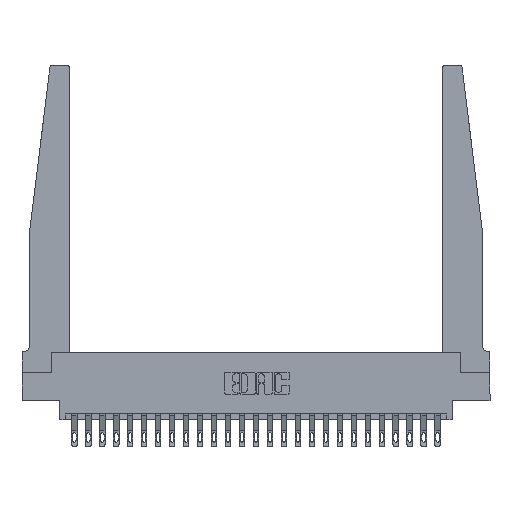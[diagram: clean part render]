
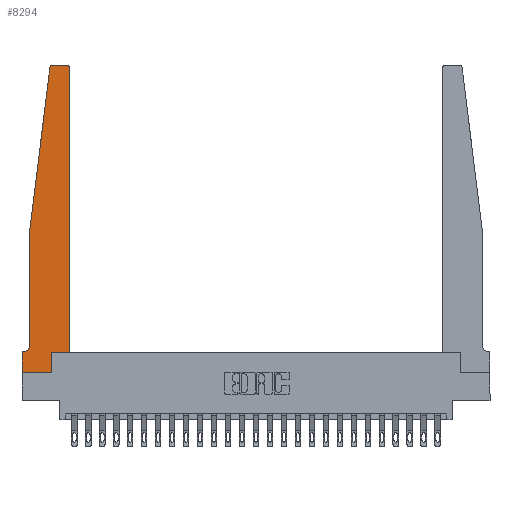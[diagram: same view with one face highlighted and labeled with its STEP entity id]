
A CAD part, top view. The second image highlights one B-rep face of the part: STEP entity #8294.
In plain terms, the highlighted planar face has unit normal (0, 0, 1).
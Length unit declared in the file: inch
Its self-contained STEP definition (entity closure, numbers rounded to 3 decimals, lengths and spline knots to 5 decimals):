
#304 = DIRECTION ( 'NONE',  ( 1., 0., 0. ) ) ;
#438 = CARTESIAN_POINT ( 'NONE',  ( 0.425, 0.18, 0.37 ) ) ;
#448 = DIRECTION ( 'NONE',  ( 1., 0., 0. ) ) ;
#450 = CARTESIAN_POINT ( 'NONE',  ( 0.065, 1.25, 0.37 ) ) ;
#496 = LINE ( 'NONE', #16148, #21478 ) ;
#976 = LINE ( 'NONE', #18656, #2612 ) ;
#987 = VERTEX_POINT ( 'NONE', #24516 ) ;
#1313 = CARTESIAN_POINT ( 'NONE',  ( 0., 0., 0.37 ) ) ;
#1725 = AXIS2_PLACEMENT_3D ( 'NONE', #16326, #2731, #22064 ) ;
#1977 = EDGE_CURVE ( 'NONE', #16019, #15077, #976, .T. ) ;
#2506 = ORIENTED_EDGE ( 'NONE', *, *, #14173, .T. ) ;
#2612 = VECTOR ( 'NONE', #22486, 39.37008 ) ;
#2731 = DIRECTION ( 'NONE',  ( 0., 0., -1. ) ) ;
#3103 = VERTEX_POINT ( 'NONE', #23181 ) ;
#3325 = CARTESIAN_POINT ( 'NONE',  ( 0.065, 1.25, 0.37 ) ) ;
#4118 = AXIS2_PLACEMENT_3D ( 'NONE', #18171, #18535, #14461 ) ;
#4523 = EDGE_CURVE ( 'NONE', #987, #17057, #13668, .T. ) ;
#4649 = VERTEX_POINT ( 'NONE', #15840 ) ;
#4900 = AXIS2_PLACEMENT_3D ( 'NONE', #19414, #17512, #448 ) ;
#5252 = EDGE_CURVE ( 'NONE', #9253, #4649, #19997, .T. ) ;
#5402 = DIRECTION ( 'NONE',  ( -1., 0., 0. ) ) ;
#5615 = DIRECTION ( 'NONE',  ( 1., 0., 0. ) ) ;
#5643 = VERTEX_POINT ( 'NONE', #18322 ) ;
#6021 = ORIENTED_EDGE ( 'NONE', *, *, #4523, .T. ) ;
#6330 = VERTEX_POINT ( 'NONE', #450 ) ;
#6332 = ORIENTED_EDGE ( 'NONE', *, *, #1977, .T. ) ;
#6504 = EDGE_CURVE ( 'NONE', #3103, #10384, #11572, .T. ) ;
#6585 = AXIS2_PLACEMENT_3D ( 'NONE', #7555, #23144, #5615 ) ;
#6631 = ORIENTED_EDGE ( 'NONE', *, *, #19101, .T. ) ;
#6882 = VECTOR ( 'NONE', #19458, 39.37008 ) ;
#7091 = ORIENTED_EDGE ( 'NONE', *, *, #15475, .T. ) ;
#7186 = CARTESIAN_POINT ( 'NONE',  ( 0.425, 0.18, 0.37 ) ) ;
#7555 = CARTESIAN_POINT ( 'NONE',  ( 0.27653, 2.72, 0.37 ) ) ;
#8294 = ADVANCED_FACE ( 'NONE', ( #16136 ), #12296, .T. ) ;
#8692 = CIRCLE ( 'NONE', #1725, 0.05 ) ;
#9253 = VERTEX_POINT ( 'NONE', #22401 ) ;
#9381 = ORIENTED_EDGE ( 'NONE', *, *, #5252, .T. ) ;
#9398 = EDGE_CURVE ( 'NONE', #11589, #6330, #13097, .T. ) ;
#9650 = VECTOR ( 'NONE', #22900, 39.37008 ) ;
#10173 = ORIENTED_EDGE ( 'NONE', *, *, #10386, .T. ) ;
#10384 = VERTEX_POINT ( 'NONE', #14288 ) ;
#10386 = EDGE_CURVE ( 'NONE', #5643, #9253, #8692, .T. ) ;
#10797 = ORIENTED_EDGE ( 'NONE', *, *, #9398, .T. ) ;
#11281 = VECTOR ( 'NONE', #17853, 39.37008 ) ;
#11572 = LINE ( 'NONE', #15533, #25183 ) ;
#11589 = VERTEX_POINT ( 'NONE', #11617 ) ;
#11617 = CARTESIAN_POINT ( 'NONE',  ( 0.24675, 2.72367, 0.37 ) ) ;
#12296 = PLANE ( 'NONE',  #4118 ) ;
#12999 = ORIENTED_EDGE ( 'NONE', *, *, #25140, .T. ) ;
#13097 = LINE ( 'NONE', #3325, #6882 ) ;
#13668 = LINE ( 'NONE', #7186, #9650 ) ;
#14169 = LINE ( 'NONE', #438, #25206 ) ;
#14173 = EDGE_CURVE ( 'NONE', #17680, #16019, #496, .T. ) ;
#14231 = DIRECTION ( 'NONE',  ( 1., 0., 0. ) ) ;
#14264 = DIRECTION ( 'NONE',  ( 0., -1., 0. ) ) ;
#14288 = CARTESIAN_POINT ( 'NONE',  ( 0.27653, 2.75, 0.37 ) ) ;
#14461 = DIRECTION ( 'NONE',  ( 1., 0., 0. ) ) ;
#14935 = EDGE_CURVE ( 'NONE', #15077, #987, #14169, .T. ) ;
#15077 = VERTEX_POINT ( 'NONE', #16584 ) ;
#15475 = EDGE_CURVE ( 'NONE', #6330, #5643, #17604, .T. ) ;
#15533 = CARTESIAN_POINT ( 'NONE',  ( 0.25, 2.75, 0.37 ) ) ;
#15551 = CARTESIAN_POINT ( 'NONE',  ( 0.065, 1.25, 0.37 ) ) ;
#15803 = CARTESIAN_POINT ( 'NONE',  ( 0., 0., 0.37 ) ) ;
#15840 = CARTESIAN_POINT ( 'NONE',  ( 0., 0.1875, 0.37 ) ) ;
#16019 = VERTEX_POINT ( 'NONE', #24544 ) ;
#16136 = FACE_OUTER_BOUND ( 'NONE', #17041, .T. ) ;
#16148 = CARTESIAN_POINT ( 'NONE',  ( 0., 0., 0.37 ) ) ;
#16183 = LINE ( 'NONE', #15803, #18735 ) ;
#16193 = DIRECTION ( 'NONE',  ( -1., 0., 0. ) ) ;
#16326 = CARTESIAN_POINT ( 'NONE',  ( 0.015, 0.2375, 0.37 ) ) ;
#16584 = CARTESIAN_POINT ( 'NONE',  ( 0.2605, 0.18, 0.37 ) ) ;
#17041 = EDGE_LOOP ( 'NONE', ( #19738, #12999, #10797, #7091, #10173, #9381, #6631, #2506, #6332, #20592, #6021, #22406 ) ) ;
#17057 = VERTEX_POINT ( 'NONE', #24152 ) ;
#17512 = DIRECTION ( 'NONE',  ( 0., 0., 1. ) ) ;
#17604 = LINE ( 'NONE', #15551, #11281 ) ;
#17680 = VERTEX_POINT ( 'NONE', #1313 ) ;
#17853 = DIRECTION ( 'NONE',  ( 0., -1., 0. ) ) ;
#18102 = CARTESIAN_POINT ( 'NONE',  ( 0.065, 0.1875, 0.37 ) ) ;
#18171 = CARTESIAN_POINT ( 'NONE',  ( 0., 0.1875, 0.37 ) ) ;
#18322 = CARTESIAN_POINT ( 'NONE',  ( 0.065, 0.2375, 0.37 ) ) ;
#18535 = DIRECTION ( 'NONE',  ( 0., 0., 1. ) ) ;
#18656 = CARTESIAN_POINT ( 'NONE',  ( 0.2605, 0.18, 0.37 ) ) ;
#18735 = VECTOR ( 'NONE', #14264, 39.37008 ) ;
#19101 = EDGE_CURVE ( 'NONE', #4649, #17680, #16183, .T. ) ;
#19414 = CARTESIAN_POINT ( 'NONE',  ( 0.395, 2.72, 0.37 ) ) ;
#19458 = DIRECTION ( 'NONE',  ( -0.122, -0.992, 0. ) ) ;
#19738 = ORIENTED_EDGE ( 'NONE', *, *, #6504, .T. ) ;
#19997 = LINE ( 'NONE', #18102, #22007 ) ;
#20592 = ORIENTED_EDGE ( 'NONE', *, *, #14935, .T. ) ;
#21138 = EDGE_CURVE ( 'NONE', #17057, #3103, #22468, .T. ) ;
#21478 = VECTOR ( 'NONE', #14231, 39.37008 ) ;
#22007 = VECTOR ( 'NONE', #16193, 39.37008 ) ;
#22064 = DIRECTION ( 'NONE',  ( -1., 0., 0. ) ) ;
#22081 = CIRCLE ( 'NONE', #6585, 0.03 ) ;
#22401 = CARTESIAN_POINT ( 'NONE',  ( 0.015, 0.1875, 0.37 ) ) ;
#22406 = ORIENTED_EDGE ( 'NONE', *, *, #21138, .T. ) ;
#22468 = CIRCLE ( 'NONE', #4900, 0.03 ) ;
#22486 = DIRECTION ( 'NONE',  ( 0., 1., 0. ) ) ;
#22900 = DIRECTION ( 'NONE',  ( 0., 1., 0. ) ) ;
#23144 = DIRECTION ( 'NONE',  ( 0., 0., 1. ) ) ;
#23181 = CARTESIAN_POINT ( 'NONE',  ( 0.395, 2.75, 0.37 ) ) ;
#24152 = CARTESIAN_POINT ( 'NONE',  ( 0.425, 2.72, 0.37 ) ) ;
#24516 = CARTESIAN_POINT ( 'NONE',  ( 0.425, 0.18, 0.37 ) ) ;
#24544 = CARTESIAN_POINT ( 'NONE',  ( 0.2605, 0., 0.37 ) ) ;
#25140 = EDGE_CURVE ( 'NONE', #10384, #11589, #22081, .T. ) ;
#25183 = VECTOR ( 'NONE', #5402, 39.37008 ) ;
#25206 = VECTOR ( 'NONE', #304, 39.37008 ) ;
